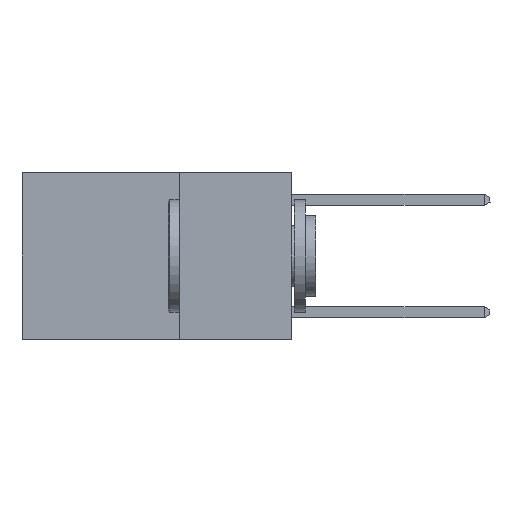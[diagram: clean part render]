
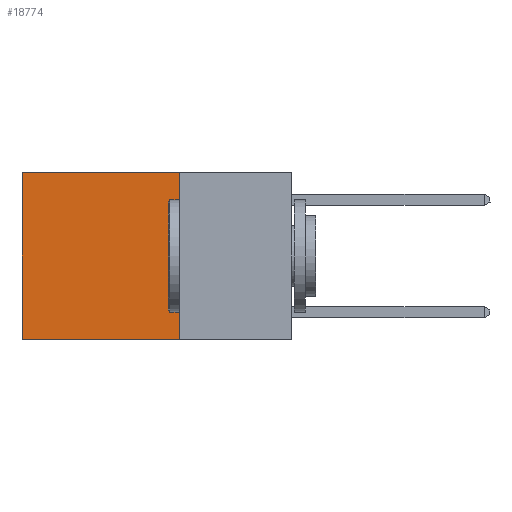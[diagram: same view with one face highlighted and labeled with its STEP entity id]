
A CAD part, left-side view. The second image highlights one B-rep face of the part: STEP entity #18774.
In plain terms, the highlighted planar face has unit normal (-1, 0, 0).
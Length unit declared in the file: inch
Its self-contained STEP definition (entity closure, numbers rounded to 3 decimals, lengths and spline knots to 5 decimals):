
#488 = VECTOR ( 'NONE', #2040, 39.37008 ) ;
#647 = VECTOR ( 'NONE', #18117, 39.37008 ) ;
#1219 = PLANE ( 'NONE',  #12943 ) ;
#1358 = CARTESIAN_POINT ( 'NONE',  ( 0.2625, 0.25, 0. ) ) ;
#1602 = CARTESIAN_POINT ( 'NONE',  ( 0.2625, 0.6, -0.37 ) ) ;
#1974 = DIRECTION ( 'NONE',  ( 0., 0., -1. ) ) ;
#2040 = DIRECTION ( 'NONE',  ( 0., 1., 0. ) ) ;
#2057 = ORIENTED_EDGE ( 'NONE', *, *, #14570, .T. ) ;
#2524 = CARTESIAN_POINT ( 'NONE',  ( 0.2625, 0.25, -0.37 ) ) ;
#2694 = VECTOR ( 'NONE', #1974, 39.37008 ) ;
#2883 = FACE_OUTER_BOUND ( 'NONE', #9605, .T. ) ;
#5361 = DIRECTION ( 'NONE',  ( 0., 1., 0. ) ) ;
#5525 = LINE ( 'NONE', #15064, #488 ) ;
#5788 = DIRECTION ( 'NONE',  ( 1., 0., 0. ) ) ;
#5870 = CARTESIAN_POINT ( 'NONE',  ( 0.2625, 0.6, 0. ) ) ;
#6492 = LINE ( 'NONE', #15625, #17356 ) ;
#7048 = VERTEX_POINT ( 'NONE', #12759 ) ;
#7221 = DIRECTION ( 'NONE',  ( 0., 0., -1. ) ) ;
#8382 = EDGE_CURVE ( 'NONE', #17358, #11086, #6492, .T. ) ;
#9605 = EDGE_LOOP ( 'NONE', ( #15079, #15348, #16175, #2057 ) ) ;
#10661 = CARTESIAN_POINT ( 'NONE',  ( 0.2625, 0.25, 0. ) ) ;
#11086 = VERTEX_POINT ( 'NONE', #1602 ) ;
#12166 = LINE ( 'NONE', #10661, #2694 ) ;
#12759 = CARTESIAN_POINT ( 'NONE',  ( 0.2625, 0.25, 0. ) ) ;
#12943 = AXIS2_PLACEMENT_3D ( 'NONE', #1358, #5788, #7221 ) ;
#12985 = EDGE_CURVE ( 'NONE', #7048, #17358, #12166, .T. ) ;
#13568 = LINE ( 'NONE', #16640, #647 ) ;
#14570 = EDGE_CURVE ( 'NONE', #7048, #14985, #5525, .T. ) ;
#14985 = VERTEX_POINT ( 'NONE', #5870 ) ;
#15064 = CARTESIAN_POINT ( 'NONE',  ( 0.2625, 0.25, 0. ) ) ;
#15079 = ORIENTED_EDGE ( 'NONE', *, *, #15937, .T. ) ;
#15348 = ORIENTED_EDGE ( 'NONE', *, *, #8382, .F. ) ;
#15625 = CARTESIAN_POINT ( 'NONE',  ( 0.2625, 0.25, -0.37 ) ) ;
#15937 = EDGE_CURVE ( 'NONE', #14985, #11086, #13568, .T. ) ;
#16175 = ORIENTED_EDGE ( 'NONE', *, *, #12985, .F. ) ;
#16640 = CARTESIAN_POINT ( 'NONE',  ( 0.2625, 0.6, 0. ) ) ;
#17356 = VECTOR ( 'NONE', #5361, 39.37008 ) ;
#17358 = VERTEX_POINT ( 'NONE', #2524 ) ;
#18117 = DIRECTION ( 'NONE',  ( 0., 0., -1. ) ) ;
#18774 = ADVANCED_FACE ( 'NONE', ( #2883 ), #1219, .F. ) ;
